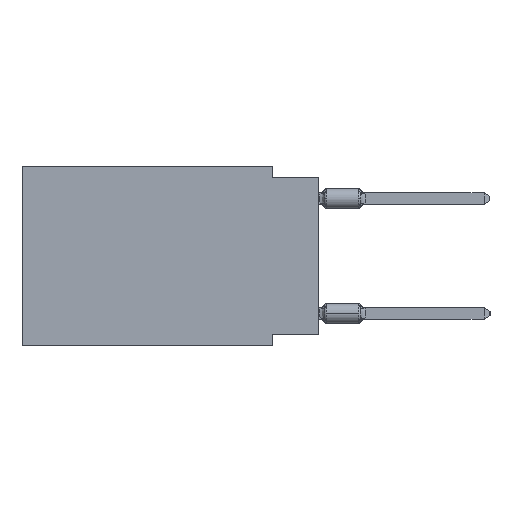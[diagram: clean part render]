
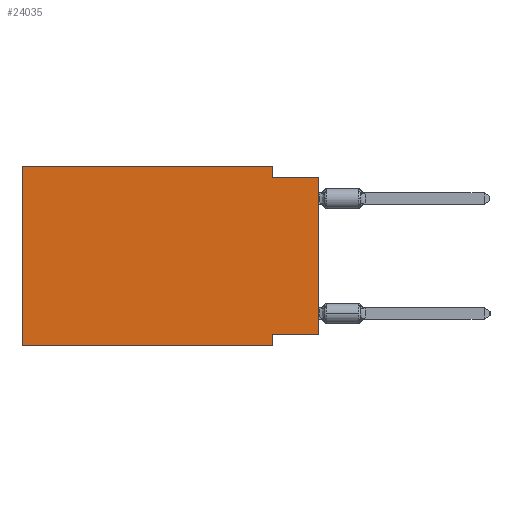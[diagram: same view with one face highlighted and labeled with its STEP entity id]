
A CAD part, left-side view. The second image highlights one B-rep face of the part: STEP entity #24035.
In plain terms, the highlighted planar face has unit normal (-1, 0, 0).
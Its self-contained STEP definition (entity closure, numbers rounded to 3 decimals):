
#89 = DIRECTION ( 'NONE',  ( 0., -1., 0. ) ) ;
#1656 = VERTEX_POINT ( 'NONE', #1801 ) ;
#1794 = DIRECTION ( 'NONE',  ( 1., 0., 0. ) ) ;
#1801 = CARTESIAN_POINT ( 'NONE',  ( 0., 2.54, -9.271 ) ) ;
#2103 = AXIS2_PLACEMENT_3D ( 'NONE', #3795, #1794, #12800 ) ;
#2152 = EDGE_CURVE ( 'NONE', #13155, #19728, #14535, .T. ) ;
#2159 = LINE ( 'NONE', #10604, #15289 ) ;
#2191 = CARTESIAN_POINT ( 'NONE',  ( 0., 2.54, 0. ) ) ;
#2580 = VERTEX_POINT ( 'NONE', #26402 ) ;
#3391 = ORIENTED_EDGE ( 'NONE', *, *, #25356, .T. ) ;
#3510 = VECTOR ( 'NONE', #23340, 1000. ) ;
#3795 = CARTESIAN_POINT ( 'NONE',  ( 0., 16.383, 0. ) ) ;
#4469 = LINE ( 'NONE', #22031, #9199 ) ;
#6164 = CARTESIAN_POINT ( 'NONE',  ( 0., 2.54, -9.906 ) ) ;
#6328 = EDGE_LOOP ( 'NONE', ( #3391, #17044, #12536, #8291, #19893, #15285, #24231, #14744 ) ) ;
#6350 = CARTESIAN_POINT ( 'NONE',  ( 0., 2.54, -0.635 ) ) ;
#6466 = LINE ( 'NONE', #2191, #8907 ) ;
#6492 = EDGE_CURVE ( 'NONE', #27823, #1656, #4469, .T. ) ;
#8291 = ORIENTED_EDGE ( 'NONE', *, *, #16437, .F. ) ;
#8494 = LINE ( 'NONE', #10931, #8949 ) ;
#8508 = VECTOR ( 'NONE', #27740, 1000. ) ;
#8642 = LINE ( 'NONE', #23912, #11241 ) ;
#8907 = VECTOR ( 'NONE', #19167, 1000. ) ;
#8949 = VECTOR ( 'NONE', #19734, 1000. ) ;
#9064 = VERTEX_POINT ( 'NONE', #13709 ) ;
#9199 = VECTOR ( 'NONE', #24464, 1000. ) ;
#9634 = LINE ( 'NONE', #14239, #27205 ) ;
#9744 = EDGE_CURVE ( 'NONE', #9064, #13155, #6466, .T. ) ;
#9929 = DIRECTION ( 'NONE',  ( 0., 0., 1. ) ) ;
#10604 = CARTESIAN_POINT ( 'NONE',  ( 0., 16.383, 0. ) ) ;
#10931 = CARTESIAN_POINT ( 'NONE',  ( 0., 16.383, -9.906 ) ) ;
#11241 = VECTOR ( 'NONE', #15277, 1000. ) ;
#12165 = VERTEX_POINT ( 'NONE', #21898 ) ;
#12536 = ORIENTED_EDGE ( 'NONE', *, *, #9744, .F. ) ;
#12800 = DIRECTION ( 'NONE',  ( 0., 0., -1. ) ) ;
#13086 = PLANE ( 'NONE',  #2103 ) ;
#13155 = VERTEX_POINT ( 'NONE', #6350 ) ;
#13709 = CARTESIAN_POINT ( 'NONE',  ( 0., 2.54, 0. ) ) ;
#13967 = CARTESIAN_POINT ( 'NONE',  ( 0., 0., -0.635 ) ) ;
#14239 = CARTESIAN_POINT ( 'NONE',  ( 0., 16.383, 0. ) ) ;
#14535 = LINE ( 'NONE', #21727, #3510 ) ;
#14744 = ORIENTED_EDGE ( 'NONE', *, *, #6492, .F. ) ;
#15277 = DIRECTION ( 'NONE',  ( 0., 0., 1. ) ) ;
#15285 = ORIENTED_EDGE ( 'NONE', *, *, #24025, .T. ) ;
#15289 = VECTOR ( 'NONE', #89, 1000. ) ;
#16437 = EDGE_CURVE ( 'NONE', #22344, #9064, #2159, .T. ) ;
#17044 = ORIENTED_EDGE ( 'NONE', *, *, #2152, .F. ) ;
#19167 = DIRECTION ( 'NONE',  ( 0., 0., -1. ) ) ;
#19728 = VERTEX_POINT ( 'NONE', #13967 ) ;
#19734 = DIRECTION ( 'NONE',  ( 0., -1., 0. ) ) ;
#19893 = ORIENTED_EDGE ( 'NONE', *, *, #28000, .F. ) ;
#21727 = CARTESIAN_POINT ( 'NONE',  ( 0., 0., -0.635 ) ) ;
#21898 = CARTESIAN_POINT ( 'NONE',  ( 0., 2.54, -9.906 ) ) ;
#22031 = CARTESIAN_POINT ( 'NONE',  ( 0., 0., -9.271 ) ) ;
#22315 = CARTESIAN_POINT ( 'NONE',  ( 0., 16.383, 0. ) ) ;
#22344 = VERTEX_POINT ( 'NONE', #22315 ) ;
#22762 = EDGE_CURVE ( 'NONE', #1656, #12165, #27599, .T. ) ;
#23340 = DIRECTION ( 'NONE',  ( 0., -1., 0. ) ) ;
#23632 = FACE_OUTER_BOUND ( 'NONE', #6328, .T. ) ;
#23912 = CARTESIAN_POINT ( 'NONE',  ( 0., 0., 0. ) ) ;
#24025 = EDGE_CURVE ( 'NONE', #2580, #12165, #8494, .T. ) ;
#24035 = ADVANCED_FACE ( 'NONE', ( #23632 ), #13086, .F. ) ;
#24231 = ORIENTED_EDGE ( 'NONE', *, *, #22762, .F. ) ;
#24464 = DIRECTION ( 'NONE',  ( 0., 1., 0. ) ) ;
#25356 = EDGE_CURVE ( 'NONE', #27823, #19728, #8642, .T. ) ;
#25795 = CARTESIAN_POINT ( 'NONE',  ( 0., 0., -9.271 ) ) ;
#26402 = CARTESIAN_POINT ( 'NONE',  ( 0., 16.383, -9.906 ) ) ;
#27205 = VECTOR ( 'NONE', #9929, 1000. ) ;
#27599 = LINE ( 'NONE', #6164, #8508 ) ;
#27740 = DIRECTION ( 'NONE',  ( 0., 0., -1. ) ) ;
#27823 = VERTEX_POINT ( 'NONE', #25795 ) ;
#28000 = EDGE_CURVE ( 'NONE', #2580, #22344, #9634, .T. ) ;
